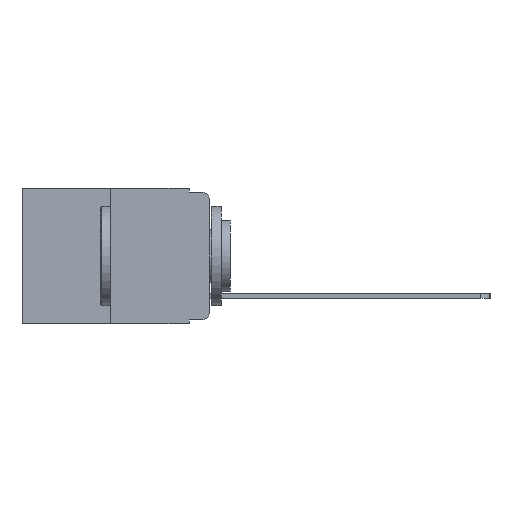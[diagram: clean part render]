
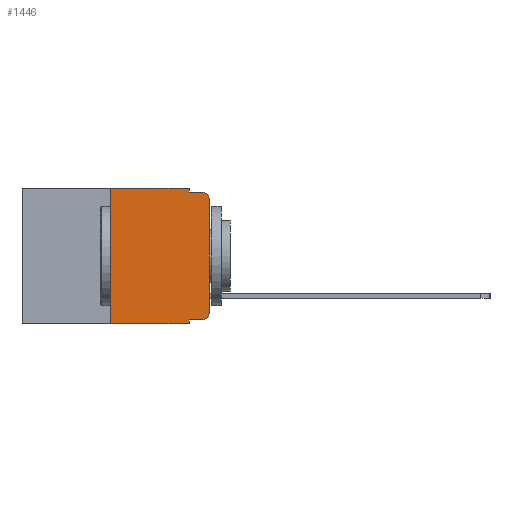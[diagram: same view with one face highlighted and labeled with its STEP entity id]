
A CAD part, left-side view. The second image highlights one B-rep face of the part: STEP entity #1446.
In plain terms, the highlighted planar face has unit normal (-1, 0, 0).
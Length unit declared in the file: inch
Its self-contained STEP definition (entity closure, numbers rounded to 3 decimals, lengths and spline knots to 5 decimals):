
#193 = PLANE ( 'NONE',  #5602 ) ;
#423 = VERTEX_POINT ( 'NONE', #4687 ) ;
#444 = ORIENTED_EDGE ( 'NONE', *, *, #4757, .T. ) ;
#481 = LINE ( 'NONE', #923, #3088 ) ;
#705 = ORIENTED_EDGE ( 'NONE', *, *, #9704, .F. ) ;
#867 = EDGE_CURVE ( 'NONE', #5574, #3766, #6947, .T. ) ;
#868 = CARTESIAN_POINT ( 'NONE',  ( 0., 0.02, -0.333 ) ) ;
#923 = CARTESIAN_POINT ( 'NONE',  ( 0., 0.473, -0.343 ) ) ;
#950 = EDGE_CURVE ( 'NONE', #3884, #423, #6086, .T. ) ;
#1145 = DIRECTION ( 'NONE',  ( 0., -1., 0. ) ) ;
#1351 = LINE ( 'NONE', #4296, #3916 ) ;
#1446 = ADVANCED_FACE ( 'NONE', ( #5247 ), #193, .F. ) ;
#1795 = EDGE_CURVE ( 'NONE', #5574, #5152, #9561, .T. ) ;
#1889 = EDGE_LOOP ( 'NONE', ( #8164, #9641, #10535, #4720, #8169, #705, #4948, #4488, #9690, #444 ) ) ;
#2214 = CARTESIAN_POINT ( 'NONE',  ( 0., 0.02, -0.01 ) ) ;
#2222 = CARTESIAN_POINT ( 'NONE',  ( 0., 0., -0.313 ) ) ;
#2836 = CARTESIAN_POINT ( 'NONE',  ( 0., 0.051, -0.01 ) ) ;
#3088 = VECTOR ( 'NONE', #6686, 39.37008 ) ;
#3235 = DIRECTION ( 'NONE',  ( -1., 0., 0. ) ) ;
#3319 = VERTEX_POINT ( 'NONE', #10341 ) ;
#3622 = AXIS2_PLACEMENT_3D ( 'NONE', #4681, #4610, #4463 ) ;
#3706 = CARTESIAN_POINT ( 'NONE',  ( 0., 0.051, 0. ) ) ;
#3766 = VERTEX_POINT ( 'NONE', #868 ) ;
#3884 = VERTEX_POINT ( 'NONE', #2222 ) ;
#3916 = VECTOR ( 'NONE', #10012, 39.37008 ) ;
#3954 = EDGE_CURVE ( 'NONE', #4920, #11022, #8177, .T. ) ;
#4192 = VECTOR ( 'NONE', #11257, 39.37008 ) ;
#4296 = CARTESIAN_POINT ( 'NONE',  ( 0., 0.473, 0. ) ) ;
#4463 = DIRECTION ( 'NONE',  ( 0., 0., -1. ) ) ;
#4488 = ORIENTED_EDGE ( 'NONE', *, *, #1795, .F. ) ;
#4610 = DIRECTION ( 'NONE',  ( -1., 0., 0. ) ) ;
#4656 = CARTESIAN_POINT ( 'NONE',  ( 0., 0.051, -0.333 ) ) ;
#4681 = CARTESIAN_POINT ( 'NONE',  ( 0., 0.02, -0.313 ) ) ;
#4687 = CARTESIAN_POINT ( 'NONE',  ( 0., 0., -0.03 ) ) ;
#4720 = ORIENTED_EDGE ( 'NONE', *, *, #5239, .F. ) ;
#4734 = DIRECTION ( 'NONE',  ( 0., 0., 1. ) ) ;
#4757 = EDGE_CURVE ( 'NONE', #3766, #3884, #5500, .T. ) ;
#4920 = VERTEX_POINT ( 'NONE', #6361 ) ;
#4948 = ORIENTED_EDGE ( 'NONE', *, *, #11848, .T. ) ;
#5152 = VERTEX_POINT ( 'NONE', #10219 ) ;
#5239 = EDGE_CURVE ( 'NONE', #3319, #4920, #6517, .T. ) ;
#5247 = FACE_OUTER_BOUND ( 'NONE', #1889, .T. ) ;
#5469 = CARTESIAN_POINT ( 'NONE',  ( 0., 0.051, -0.333 ) ) ;
#5472 = VECTOR ( 'NONE', #7593, 39.37008 ) ;
#5500 = CIRCLE ( 'NONE', #3622, 0.02 ) ;
#5574 = VERTEX_POINT ( 'NONE', #4656 ) ;
#5602 = AXIS2_PLACEMENT_3D ( 'NONE', #8606, #5715, #10783 ) ;
#5649 = VECTOR ( 'NONE', #1145, 39.37008 ) ;
#5715 = DIRECTION ( 'NONE',  ( 1., 0., 0. ) ) ;
#5745 = CARTESIAN_POINT ( 'NONE',  ( 0., 0., 0. ) ) ;
#5967 = VERTEX_POINT ( 'NONE', #8125 ) ;
#6086 = LINE ( 'NONE', #5745, #5472 ) ;
#6361 = CARTESIAN_POINT ( 'NONE',  ( 0., 0.051, -0.01 ) ) ;
#6517 = LINE ( 'NONE', #6679, #11256 ) ;
#6610 = DIRECTION ( 'NONE',  ( 0., 0., -1. ) ) ;
#6660 = VECTOR ( 'NONE', #9948, 39.37008 ) ;
#6679 = CARTESIAN_POINT ( 'NONE',  ( 0., 0.051, 0. ) ) ;
#6686 = DIRECTION ( 'NONE',  ( 0., -1., 0. ) ) ;
#6947 = LINE ( 'NONE', #5469, #6660 ) ;
#7004 = CARTESIAN_POINT ( 'NONE',  ( 0., 0.25, 0. ) ) ;
#7593 = DIRECTION ( 'NONE',  ( 0., 0., 1. ) ) ;
#8069 = VECTOR ( 'NONE', #4734, 39.37008 ) ;
#8125 = CARTESIAN_POINT ( 'NONE',  ( 0., 0.25, -0.343 ) ) ;
#8164 = ORIENTED_EDGE ( 'NONE', *, *, #950, .T. ) ;
#8169 = ORIENTED_EDGE ( 'NONE', *, *, #8743, .F. ) ;
#8177 = LINE ( 'NONE', #2836, #5649 ) ;
#8606 = CARTESIAN_POINT ( 'NONE',  ( 0., 0.473, 0. ) ) ;
#8743 = EDGE_CURVE ( 'NONE', #11485, #3319, #1351, .T. ) ;
#8940 = CARTESIAN_POINT ( 'NONE',  ( 0., 0.02, -0.03 ) ) ;
#9561 = LINE ( 'NONE', #3706, #4192 ) ;
#9641 = ORIENTED_EDGE ( 'NONE', *, *, #10572, .T. ) ;
#9690 = ORIENTED_EDGE ( 'NONE', *, *, #867, .T. ) ;
#9704 = EDGE_CURVE ( 'NONE', #5967, #11485, #10585, .T. ) ;
#9896 = DIRECTION ( 'NONE',  ( 0., 0., -1. ) ) ;
#9948 = DIRECTION ( 'NONE',  ( 0., -1., 0. ) ) ;
#10012 = DIRECTION ( 'NONE',  ( 0., -1., 0. ) ) ;
#10219 = CARTESIAN_POINT ( 'NONE',  ( 0., 0.051, -0.343 ) ) ;
#10341 = CARTESIAN_POINT ( 'NONE',  ( 0., 0.051, 0. ) ) ;
#10398 = AXIS2_PLACEMENT_3D ( 'NONE', #8940, #3235, #9896 ) ;
#10435 = CARTESIAN_POINT ( 'NONE',  ( 0., 0.25, 0. ) ) ;
#10535 = ORIENTED_EDGE ( 'NONE', *, *, #3954, .F. ) ;
#10572 = EDGE_CURVE ( 'NONE', #423, #11022, #11136, .T. ) ;
#10585 = LINE ( 'NONE', #10435, #8069 ) ;
#10783 = DIRECTION ( 'NONE',  ( 0., 0., -1. ) ) ;
#11022 = VERTEX_POINT ( 'NONE', #2214 ) ;
#11136 = CIRCLE ( 'NONE', #10398, 0.02 ) ;
#11256 = VECTOR ( 'NONE', #6610, 39.37008 ) ;
#11257 = DIRECTION ( 'NONE',  ( 0., 0., -1. ) ) ;
#11485 = VERTEX_POINT ( 'NONE', #7004 ) ;
#11848 = EDGE_CURVE ( 'NONE', #5967, #5152, #481, .T. ) ;
